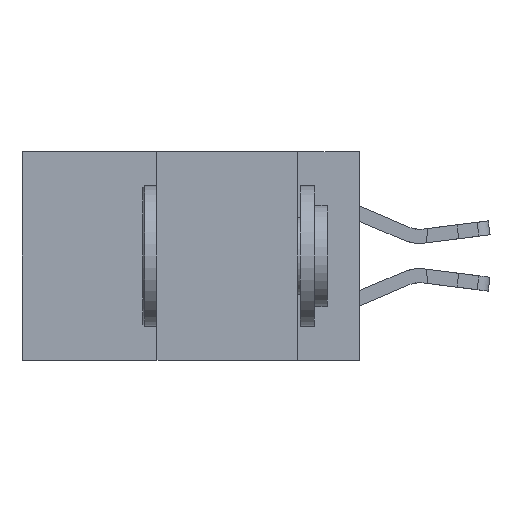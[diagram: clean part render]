
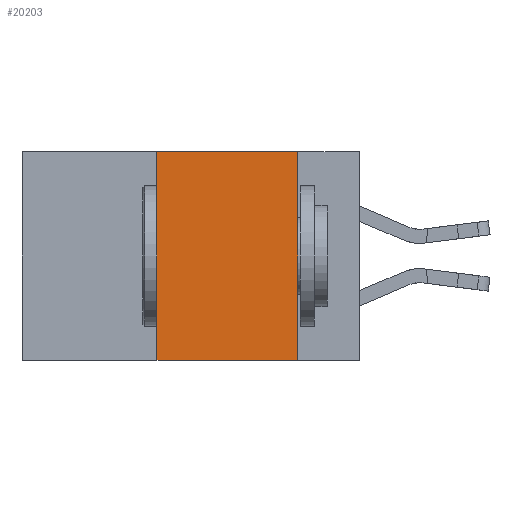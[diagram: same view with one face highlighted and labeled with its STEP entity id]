
A CAD part, left-side view. The second image highlights one B-rep face of the part: STEP entity #20203.
In plain terms, the highlighted planar face has unit normal (-1, 0, 0).
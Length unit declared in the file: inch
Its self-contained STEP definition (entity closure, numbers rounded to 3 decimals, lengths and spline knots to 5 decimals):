
#149 = VECTOR ( 'NONE', #9214, 39.37008 ) ;
#894 = CARTESIAN_POINT ( 'NONE',  ( 0., 0.36, -0.37 ) ) ;
#913 = VECTOR ( 'NONE', #9038, 39.37008 ) ;
#1380 = CARTESIAN_POINT ( 'NONE',  ( 0., 0.6, 0. ) ) ;
#2083 = CARTESIAN_POINT ( 'NONE',  ( 0., 0.36, 0. ) ) ;
#2234 = VERTEX_POINT ( 'NONE', #894 ) ;
#3494 = CARTESIAN_POINT ( 'NONE',  ( 0., 0.6, 0. ) ) ;
#4614 = ORIENTED_EDGE ( 'NONE', *, *, #10333, .T. ) ;
#4854 = CARTESIAN_POINT ( 'NONE',  ( 0., 0.6, -0.37 ) ) ;
#4881 = LINE ( 'NONE', #1380, #16982 ) ;
#5080 = LINE ( 'NONE', #18648, #913 ) ;
#5297 = ORIENTED_EDGE ( 'NONE', *, *, #5467, .F. ) ;
#5349 = LINE ( 'NONE', #9145, #149 ) ;
#5467 = EDGE_CURVE ( 'NONE', #2234, #18271, #5349, .T. ) ;
#6296 = ORIENTED_EDGE ( 'NONE', *, *, #20006, .F. ) ;
#7118 = CARTESIAN_POINT ( 'NONE',  ( 0., 0.11, -0.37 ) ) ;
#8370 = CARTESIAN_POINT ( 'NONE',  ( 0., 0.11, 0. ) ) ;
#9038 = DIRECTION ( 'NONE',  ( 0., 0., -1. ) ) ;
#9145 = CARTESIAN_POINT ( 'NONE',  ( 0., 0.36, 0. ) ) ;
#9214 = DIRECTION ( 'NONE',  ( 0., 0., 1. ) ) ;
#9377 = EDGE_CURVE ( 'NONE', #18271, #12599, #4881, .T. ) ;
#9615 = EDGE_LOOP ( 'NONE', ( #6296, #19535, #5297, #4614 ) ) ;
#10333 = EDGE_CURVE ( 'NONE', #2234, #15867, #11743, .T. ) ;
#11421 = DIRECTION ( 'NONE',  ( 1., 0., 0. ) ) ;
#11743 = LINE ( 'NONE', #4854, #12254 ) ;
#12254 = VECTOR ( 'NONE', #17666, 39.37008 ) ;
#12599 = VERTEX_POINT ( 'NONE', #8370 ) ;
#12959 = PLANE ( 'NONE',  #16572 ) ;
#15420 = DIRECTION ( 'NONE',  ( 0., -1., 0. ) ) ;
#15867 = VERTEX_POINT ( 'NONE', #7118 ) ;
#16572 = AXIS2_PLACEMENT_3D ( 'NONE', #3494, #11421, #19328 ) ;
#16982 = VECTOR ( 'NONE', #15420, 39.37008 ) ;
#17666 = DIRECTION ( 'NONE',  ( 0., -1., 0. ) ) ;
#18271 = VERTEX_POINT ( 'NONE', #2083 ) ;
#18396 = FACE_OUTER_BOUND ( 'NONE', #9615, .T. ) ;
#18648 = CARTESIAN_POINT ( 'NONE',  ( 0., 0.11, 0. ) ) ;
#19328 = DIRECTION ( 'NONE',  ( 0., 0., -1. ) ) ;
#19535 = ORIENTED_EDGE ( 'NONE', *, *, #9377, .F. ) ;
#20006 = EDGE_CURVE ( 'NONE', #12599, #15867, #5080, .T. ) ;
#20203 = ADVANCED_FACE ( 'NONE', ( #18396 ), #12959, .F. ) ;
